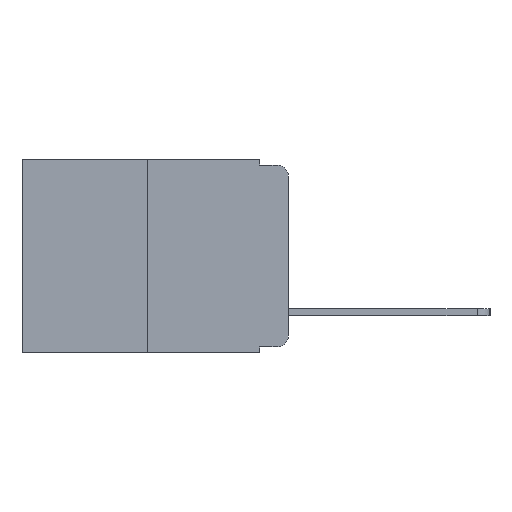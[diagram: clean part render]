
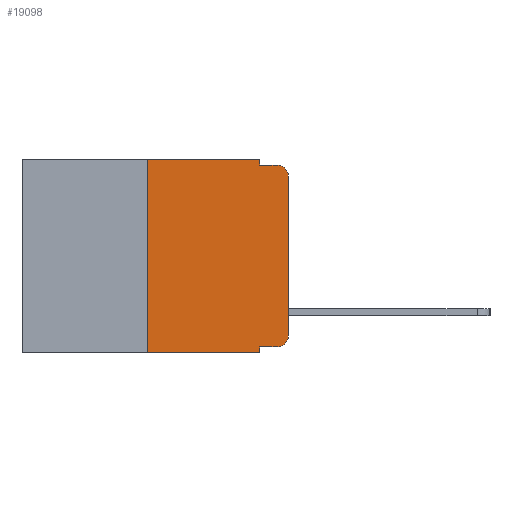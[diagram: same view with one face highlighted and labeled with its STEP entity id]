
A CAD part, left-side view. The second image highlights one B-rep face of the part: STEP entity #19098.
In plain terms, the highlighted planar face has unit normal (-1, 0, 0).
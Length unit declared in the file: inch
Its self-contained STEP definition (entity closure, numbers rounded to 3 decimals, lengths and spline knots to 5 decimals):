
#21 = VECTOR ( 'NONE', #17826, 39.37008 ) ;
#150 = VECTOR ( 'NONE', #18981, 39.37008 ) ;
#1358 = DIRECTION ( 'NONE',  ( 0., 0., -1. ) ) ;
#1443 = DIRECTION ( 'NONE',  ( 0., -1., 0. ) ) ;
#1499 = CARTESIAN_POINT ( 'NONE',  ( 0., 0.02, -0.03 ) ) ;
#1524 = ORIENTED_EDGE ( 'NONE', *, *, #9911, .F. ) ;
#2562 = VECTOR ( 'NONE', #17845, 39.37008 ) ;
#2572 = AXIS2_PLACEMENT_3D ( 'NONE', #9276, #20914, #10998 ) ;
#3181 = DIRECTION ( 'NONE',  ( 0., 0., -1. ) ) ;
#3383 = PLANE ( 'NONE',  #9593 ) ;
#3613 = VECTOR ( 'NONE', #19720, 39.37008 ) ;
#4035 = CARTESIAN_POINT ( 'NONE',  ( 0., 0.051, -0.333 ) ) ;
#4136 = LINE ( 'NONE', #14708, #3613 ) ;
#4481 = VECTOR ( 'NONE', #12029, 39.37008 ) ;
#4544 = LINE ( 'NONE', #21382, #7448 ) ;
#4594 = EDGE_CURVE ( 'NONE', #9439, #20018, #16929, .T. ) ;
#5098 = VERTEX_POINT ( 'NONE', #18323 ) ;
#5191 = ORIENTED_EDGE ( 'NONE', *, *, #6578, .T. ) ;
#5362 = CARTESIAN_POINT ( 'NONE',  ( 0., 0.473, -0.343 ) ) ;
#6250 = CARTESIAN_POINT ( 'NONE',  ( 0., 0.473, 0. ) ) ;
#6578 = EDGE_CURVE ( 'NONE', #7599, #15394, #9604, .T. ) ;
#6762 = DIRECTION ( 'NONE',  ( 1., 0., 0. ) ) ;
#6771 = ORIENTED_EDGE ( 'NONE', *, *, #17682, .T. ) ;
#7275 = VERTEX_POINT ( 'NONE', #10277 ) ;
#7448 = VECTOR ( 'NONE', #1443, 39.37008 ) ;
#7581 = VERTEX_POINT ( 'NONE', #9371 ) ;
#7599 = VERTEX_POINT ( 'NONE', #13039 ) ;
#7650 = VECTOR ( 'NONE', #1358, 39.37008 ) ;
#7927 = CARTESIAN_POINT ( 'NONE',  ( 0., 0.25, 0. ) ) ;
#8102 = VECTOR ( 'NONE', #8706, 39.37008 ) ;
#8706 = DIRECTION ( 'NONE',  ( 0., -1., 0. ) ) ;
#8790 = EDGE_CURVE ( 'NONE', #14455, #7599, #4544, .T. ) ;
#9276 = CARTESIAN_POINT ( 'NONE',  ( 0., 0.02, -0.313 ) ) ;
#9346 = ORIENTED_EDGE ( 'NONE', *, *, #12166, .F. ) ;
#9371 = CARTESIAN_POINT ( 'NONE',  ( 0., 0.25, 0. ) ) ;
#9408 = CIRCLE ( 'NONE', #9987, 0.02 ) ;
#9431 = LINE ( 'NONE', #6250, #21 ) ;
#9439 = VERTEX_POINT ( 'NONE', #9831 ) ;
#9593 = AXIS2_PLACEMENT_3D ( 'NONE', #16677, #6762, #18337 ) ;
#9604 = CIRCLE ( 'NONE', #2572, 0.02 ) ;
#9831 = CARTESIAN_POINT ( 'NONE',  ( 0., 0.25, -0.343 ) ) ;
#9911 = EDGE_CURVE ( 'NONE', #14455, #20018, #13125, .T. ) ;
#9987 = AXIS2_PLACEMENT_3D ( 'NONE', #1499, #13182, #3181 ) ;
#10277 = CARTESIAN_POINT ( 'NONE',  ( 0., 0.051, 0. ) ) ;
#10507 = EDGE_CURVE ( 'NONE', #7581, #7275, #9431, .T. ) ;
#10954 = ORIENTED_EDGE ( 'NONE', *, *, #8790, .T. ) ;
#10998 = DIRECTION ( 'NONE',  ( 0., 0., -1. ) ) ;
#11722 = ORIENTED_EDGE ( 'NONE', *, *, #16568, .T. ) ;
#12029 = DIRECTION ( 'NONE',  ( 0., -1., 0. ) ) ;
#12166 = EDGE_CURVE ( 'NONE', #9439, #7581, #19227, .T. ) ;
#12240 = CARTESIAN_POINT ( 'NONE',  ( 0., 0., -0.03 ) ) ;
#13039 = CARTESIAN_POINT ( 'NONE',  ( 0., 0.02, -0.333 ) ) ;
#13125 = LINE ( 'NONE', #21293, #7650 ) ;
#13182 = DIRECTION ( 'NONE',  ( -1., 0., 0. ) ) ;
#13274 = EDGE_CURVE ( 'NONE', #7275, #14831, #14006, .T. ) ;
#14006 = LINE ( 'NONE', #17292, #150 ) ;
#14314 = ORIENTED_EDGE ( 'NONE', *, *, #4594, .T. ) ;
#14455 = VERTEX_POINT ( 'NONE', #4035 ) ;
#14708 = CARTESIAN_POINT ( 'NONE',  ( 0., 0., 0. ) ) ;
#14831 = VERTEX_POINT ( 'NONE', #16592 ) ;
#15043 = FACE_OUTER_BOUND ( 'NONE', #15247, .T. ) ;
#15247 = EDGE_LOOP ( 'NONE', ( #6771, #11722, #20529, #17131, #17650, #9346, #14314, #1524, #10954, #5191 ) ) ;
#15394 = VERTEX_POINT ( 'NONE', #19991 ) ;
#15489 = EDGE_CURVE ( 'NONE', #14831, #5098, #17734, .T. ) ;
#16568 = EDGE_CURVE ( 'NONE', #18649, #5098, #9408, .T. ) ;
#16592 = CARTESIAN_POINT ( 'NONE',  ( 0., 0.051, -0.01 ) ) ;
#16677 = CARTESIAN_POINT ( 'NONE',  ( 0., 0.473, 0. ) ) ;
#16929 = LINE ( 'NONE', #5362, #8102 ) ;
#17131 = ORIENTED_EDGE ( 'NONE', *, *, #13274, .F. ) ;
#17292 = CARTESIAN_POINT ( 'NONE',  ( 0., 0.051, 0. ) ) ;
#17650 = ORIENTED_EDGE ( 'NONE', *, *, #10507, .F. ) ;
#17682 = EDGE_CURVE ( 'NONE', #15394, #18649, #4136, .T. ) ;
#17734 = LINE ( 'NONE', #18599, #4481 ) ;
#17826 = DIRECTION ( 'NONE',  ( 0., -1., 0. ) ) ;
#17845 = DIRECTION ( 'NONE',  ( 0., 0., 1. ) ) ;
#18323 = CARTESIAN_POINT ( 'NONE',  ( 0., 0.02, -0.01 ) ) ;
#18337 = DIRECTION ( 'NONE',  ( 0., 0., -1. ) ) ;
#18599 = CARTESIAN_POINT ( 'NONE',  ( 0., 0.051, -0.01 ) ) ;
#18649 = VERTEX_POINT ( 'NONE', #12240 ) ;
#18981 = DIRECTION ( 'NONE',  ( 0., 0., -1. ) ) ;
#19098 = ADVANCED_FACE ( 'NONE', ( #15043 ), #3383, .F. ) ;
#19227 = LINE ( 'NONE', #7927, #2562 ) ;
#19720 = DIRECTION ( 'NONE',  ( 0., 0., 1. ) ) ;
#19991 = CARTESIAN_POINT ( 'NONE',  ( 0., 0., -0.313 ) ) ;
#20018 = VERTEX_POINT ( 'NONE', #20894 ) ;
#20529 = ORIENTED_EDGE ( 'NONE', *, *, #15489, .F. ) ;
#20894 = CARTESIAN_POINT ( 'NONE',  ( 0., 0.051, -0.343 ) ) ;
#20914 = DIRECTION ( 'NONE',  ( -1., 0., 0. ) ) ;
#21293 = CARTESIAN_POINT ( 'NONE',  ( 0., 0.051, 0. ) ) ;
#21382 = CARTESIAN_POINT ( 'NONE',  ( 0., 0.051, -0.333 ) ) ;
